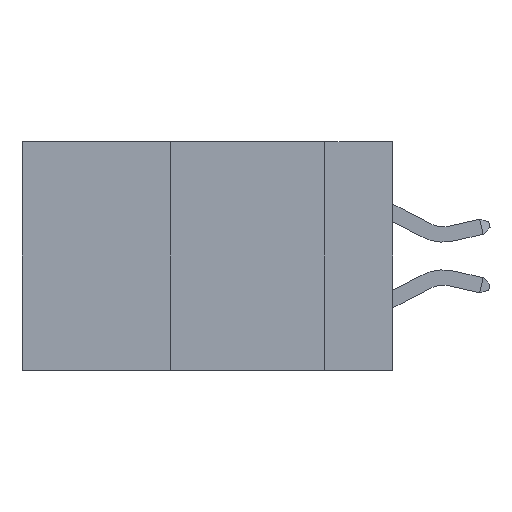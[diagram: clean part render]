
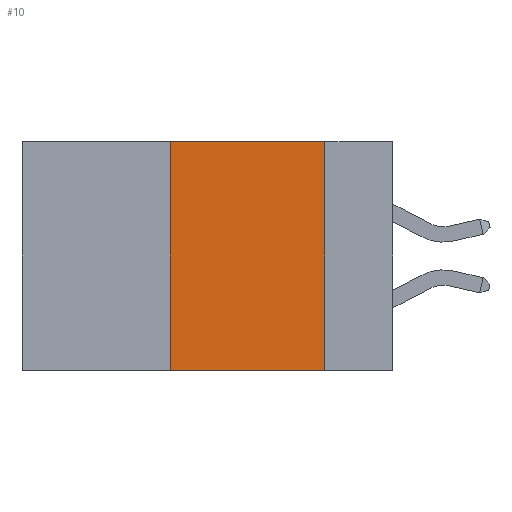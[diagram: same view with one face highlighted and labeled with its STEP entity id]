
A CAD part, left-side view. The second image highlights one B-rep face of the part: STEP entity #10.
In plain terms, the highlighted planar face has unit normal (-1, 0, 0).
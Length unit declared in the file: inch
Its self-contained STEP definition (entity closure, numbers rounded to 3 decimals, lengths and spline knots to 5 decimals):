
#10 = ADVANCED_FACE ( 'NONE', ( #5153 ), #5528, .F. ) ;
#1080 = VERTEX_POINT ( 'NONE', #1238 ) ;
#1137 = LINE ( 'NONE', #4975, #4837 ) ;
#1238 = CARTESIAN_POINT ( 'NONE',  ( 0., 0.36, -0.37 ) ) ;
#1380 = VECTOR ( 'NONE', #2755, 39.37008 ) ;
#1880 = EDGE_CURVE ( 'NONE', #2962, #6934, #7540, .T. ) ;
#2755 = DIRECTION ( 'NONE',  ( 0., 0., 1. ) ) ;
#2962 = VERTEX_POINT ( 'NONE', #4416 ) ;
#2997 = AXIS2_PLACEMENT_3D ( 'NONE', #4949, #7539, #3051 ) ;
#3051 = DIRECTION ( 'NONE',  ( 0., 0., -1. ) ) ;
#3492 = CARTESIAN_POINT ( 'NONE',  ( 0., 0.36, 0. ) ) ;
#3647 = EDGE_CURVE ( 'NONE', #5654, #2962, #5321, .T. ) ;
#4416 = CARTESIAN_POINT ( 'NONE',  ( 0., 0.11, 0. ) ) ;
#4837 = VECTOR ( 'NONE', #5669, 39.37008 ) ;
#4949 = CARTESIAN_POINT ( 'NONE',  ( 0., 0.6, 0. ) ) ;
#4975 = CARTESIAN_POINT ( 'NONE',  ( 0., 0.6, -0.37 ) ) ;
#5109 = VECTOR ( 'NONE', #5442, 39.37008 ) ;
#5153 = FACE_OUTER_BOUND ( 'NONE', #8435, .T. ) ;
#5321 = LINE ( 'NONE', #5390, #5109 ) ;
#5390 = CARTESIAN_POINT ( 'NONE',  ( 0., 0.6, 0. ) ) ;
#5442 = DIRECTION ( 'NONE',  ( 0., -1., 0. ) ) ;
#5528 = PLANE ( 'NONE',  #2997 ) ;
#5654 = VERTEX_POINT ( 'NONE', #6580 ) ;
#5669 = DIRECTION ( 'NONE',  ( 0., -1., 0. ) ) ;
#5719 = ORIENTED_EDGE ( 'NONE', *, *, #3647, .F. ) ;
#6380 = DIRECTION ( 'NONE',  ( 0., 0., -1. ) ) ;
#6580 = CARTESIAN_POINT ( 'NONE',  ( 0., 0.36, 0. ) ) ;
#6934 = VERTEX_POINT ( 'NONE', #7922 ) ;
#7314 = VECTOR ( 'NONE', #6380, 39.37008 ) ;
#7340 = LINE ( 'NONE', #3492, #1380 ) ;
#7345 = CARTESIAN_POINT ( 'NONE',  ( 0., 0.11, 0. ) ) ;
#7472 = ORIENTED_EDGE ( 'NONE', *, *, #8996, .F. ) ;
#7539 = DIRECTION ( 'NONE',  ( 1., 0., 0. ) ) ;
#7540 = LINE ( 'NONE', #7345, #7314 ) ;
#7589 = ORIENTED_EDGE ( 'NONE', *, *, #9042, .T. ) ;
#7876 = ORIENTED_EDGE ( 'NONE', *, *, #1880, .F. ) ;
#7922 = CARTESIAN_POINT ( 'NONE',  ( 0., 0.11, -0.37 ) ) ;
#8435 = EDGE_LOOP ( 'NONE', ( #7876, #5719, #7472, #7589 ) ) ;
#8996 = EDGE_CURVE ( 'NONE', #1080, #5654, #7340, .T. ) ;
#9042 = EDGE_CURVE ( 'NONE', #1080, #6934, #1137, .T. ) ;
